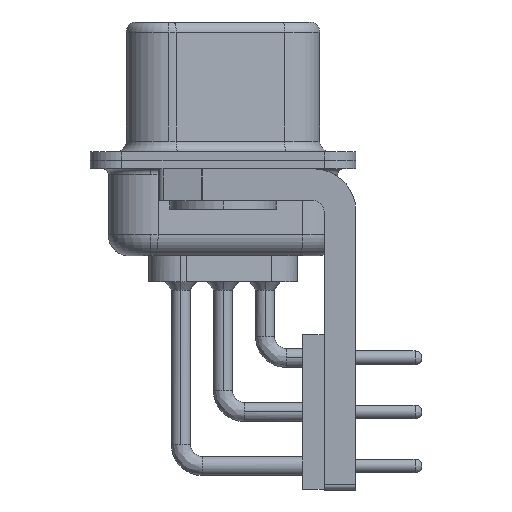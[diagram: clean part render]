
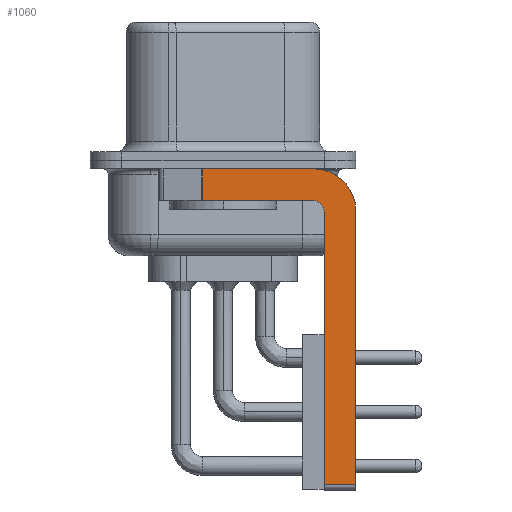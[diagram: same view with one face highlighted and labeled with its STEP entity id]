
A CAD part, left-side view. The second image highlights one B-rep face of the part: STEP entity #1060.
In plain terms, the highlighted planar face has unit normal (-1, 0, 0).
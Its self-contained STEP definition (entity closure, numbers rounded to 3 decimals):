
#245 = DIRECTION ( 'NONE',  ( -1., 0., 0. ) ) ;
#250 = DIRECTION ( 'NONE',  ( 0., 0., 1. ) ) ;
#319 = LINE ( 'NONE', #3367, #1324 ) ;
#374 = DIRECTION ( 'NONE',  ( 0., 0., -1. ) ) ;
#924 = EDGE_CURVE ( 'NONE', #10504, #36767, #14488, .T. ) ;
#1060 = ADVANCED_FACE ( 'NONE', ( #2604 ), #10896, .F. ) ;
#1324 = VECTOR ( 'NONE', #4497, 1000. ) ;
#1583 = CARTESIAN_POINT ( 'NONE',  ( -2.9, 0.978, -1.9 ) ) ;
#1650 = CARTESIAN_POINT ( 'NONE',  ( -2.9, 0.978, -0.4 ) ) ;
#2131 = DIRECTION ( 'NONE',  ( 0., 0., -1. ) ) ;
#2604 = FACE_OUTER_BOUND ( 'NONE', #20408, .T. ) ;
#3367 = CARTESIAN_POINT ( 'NONE',  ( -2.9, -4.25, -1.9 ) ) ;
#3842 = VERTEX_POINT ( 'NONE', #13668 ) ;
#4497 = DIRECTION ( 'NONE',  ( 0., 1., 0. ) ) ;
#5336 = EDGE_CURVE ( 'NONE', #3842, #36767, #319, .T. ) ;
#5742 = LINE ( 'NONE', #11406, #20827 ) ;
#5950 = EDGE_CURVE ( 'NONE', #18638, #3842, #8079, .T. ) ;
#6474 = CARTESIAN_POINT ( 'NONE',  ( -2.9, -4.25, -2.4 ) ) ;
#7050 = DIRECTION ( 'NONE',  ( 0., -1., 0. ) ) ;
#7685 = AXIS2_PLACEMENT_3D ( 'NONE', #6474, #12503, #16830 ) ;
#8079 = CIRCLE ( 'NONE', #35080, 0.5 ) ;
#8178 = CARTESIAN_POINT ( 'NONE',  ( -2.9, -4.25, -2.4 ) ) ;
#9463 = VECTOR ( 'NONE', #32560, 1000. ) ;
#9811 = CIRCLE ( 'NONE', #27210, 2. ) ;
#10342 = EDGE_CURVE ( 'NONE', #16254, #26834, #31511, .T. ) ;
#10504 = VERTEX_POINT ( 'NONE', #1650 ) ;
#10896 = PLANE ( 'NONE',  #7685 ) ;
#11165 = DIRECTION ( 'NONE',  ( 0., 0., -1. ) ) ;
#11371 = ORIENTED_EDGE ( 'NONE', *, *, #18571, .F. ) ;
#11406 = CARTESIAN_POINT ( 'NONE',  ( -2.9, -4.75, -15.5 ) ) ;
#12503 = DIRECTION ( 'NONE',  ( 1., 0., 0. ) ) ;
#13543 = ORIENTED_EDGE ( 'NONE', *, *, #15508, .F. ) ;
#13668 = CARTESIAN_POINT ( 'NONE',  ( -2.9, -4.25, -1.9 ) ) ;
#14147 = ORIENTED_EDGE ( 'NONE', *, *, #22162, .F. ) ;
#14386 = ORIENTED_EDGE ( 'NONE', *, *, #37670, .F. ) ;
#14479 = DIRECTION ( 'NONE',  ( 0., 0., 1. ) ) ;
#14488 = LINE ( 'NONE', #1583, #36344 ) ;
#15508 = EDGE_CURVE ( 'NONE', #17545, #26834, #38403, .T. ) ;
#15611 = VECTOR ( 'NONE', #7050, 1000. ) ;
#16254 = VERTEX_POINT ( 'NONE', #22786 ) ;
#16830 = DIRECTION ( 'NONE',  ( 0., 0., -1. ) ) ;
#17013 = CARTESIAN_POINT ( 'NONE',  ( -2.9, -4.25, -2.4 ) ) ;
#17545 = VERTEX_POINT ( 'NONE', #27017 ) ;
#18571 = EDGE_CURVE ( 'NONE', #25798, #17545, #9811, .T. ) ;
#18598 = CARTESIAN_POINT ( 'NONE',  ( -2.9, -6.25, -2.4 ) ) ;
#18638 = VERTEX_POINT ( 'NONE', #20411 ) ;
#19155 = CARTESIAN_POINT ( 'NONE',  ( -2.9, -4.25, -15.25 ) ) ;
#20290 = CARTESIAN_POINT ( 'NONE',  ( -2.9, -6.25, -15.25 ) ) ;
#20408 = EDGE_LOOP ( 'NONE', ( #14386, #25209, #38887, #27691, #14147, #34124, #13543, #11371 ) ) ;
#20411 = CARTESIAN_POINT ( 'NONE',  ( -2.9, -4.75, -2.4 ) ) ;
#20608 = CARTESIAN_POINT ( 'NONE',  ( -2.9, 3., -0.4 ) ) ;
#20827 = VECTOR ( 'NONE', #14479, 1000. ) ;
#22162 = EDGE_CURVE ( 'NONE', #16254, #18638, #5742, .T. ) ;
#22786 = CARTESIAN_POINT ( 'NONE',  ( -2.9, -4.75, -15.25 ) ) ;
#25209 = ORIENTED_EDGE ( 'NONE', *, *, #924, .T. ) ;
#25498 = LINE ( 'NONE', #20608, #9463 ) ;
#25798 = VERTEX_POINT ( 'NONE', #33326 ) ;
#26834 = VERTEX_POINT ( 'NONE', #20290 ) ;
#27017 = CARTESIAN_POINT ( 'NONE',  ( -2.9, -6.25, -2.4 ) ) ;
#27210 = AXIS2_PLACEMENT_3D ( 'NONE', #8178, #29141, #11165 ) ;
#27691 = ORIENTED_EDGE ( 'NONE', *, *, #5950, .F. ) ;
#29141 = DIRECTION ( 'NONE',  ( 1., 0., 0. ) ) ;
#30570 = VECTOR ( 'NONE', #374, 1000. ) ;
#31511 = LINE ( 'NONE', #19155, #15611 ) ;
#32560 = DIRECTION ( 'NONE',  ( 0., -1., 0. ) ) ;
#33326 = CARTESIAN_POINT ( 'NONE',  ( -2.9, -4.25, -0.4 ) ) ;
#33511 = CARTESIAN_POINT ( 'NONE',  ( -2.9, 0.978, -1.9 ) ) ;
#34124 = ORIENTED_EDGE ( 'NONE', *, *, #10342, .T. ) ;
#35080 = AXIS2_PLACEMENT_3D ( 'NONE', #17013, #245, #250 ) ;
#36344 = VECTOR ( 'NONE', #2131, 1000. ) ;
#36767 = VERTEX_POINT ( 'NONE', #33511 ) ;
#37670 = EDGE_CURVE ( 'NONE', #10504, #25798, #25498, .T. ) ;
#38403 = LINE ( 'NONE', #18598, #30570 ) ;
#38887 = ORIENTED_EDGE ( 'NONE', *, *, #5336, .F. ) ;
